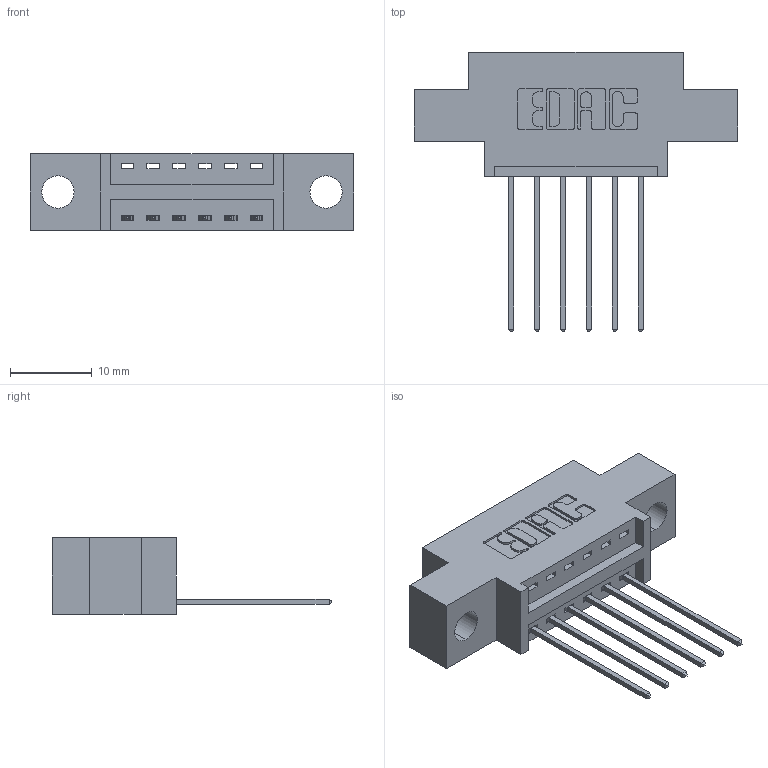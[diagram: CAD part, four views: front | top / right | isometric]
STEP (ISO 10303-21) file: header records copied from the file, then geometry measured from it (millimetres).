
FILE_DESCRIPTION (( 'STEP AP203' ), '1' );
FILE_NAME ('346-006-541-604.STEP', '2022-05-04T19:02:00', ( '' ), ( '' ), 'SwSTEP 2.0', 'SolidWorks 2020', '' );
FILE_SCHEMA (( 'CONFIG_CONTROL_DESIGN' ));
Length unit declared in the file: inch
Products named in the file (3): 345-292-001_345-293-141; 346 Part_0.170 Offset - 0.156 Dia-TH; 346-006-541-604
Assembly tree (7 placements, depth 2):
  346-006-541-604
    346 Part_0.170 Offset - 0.156 Dia-TH
    345-292-001_345-293-141  x6
Bounding box: 39.62 x 34.29 x 9.4 mm (x, y, z)
Volume: 3304.1 mm3; surface area: 3857.1 mm2
Topology: 7 solids, 7 shells, 488 faces, 1433 edges, 946 vertices
Faces by surface type: plane 334, cylinder 154
Entity records: 9139 total; most frequent: CARTESIAN_POINT 1588, ORIENTED_EDGE 1526, DIRECTION 1443, EDGE_CURVE 763, VECTOR 607, LINE 607, VERTEX_POINT 506, AXIS2_PLACEMENT_3D 418
